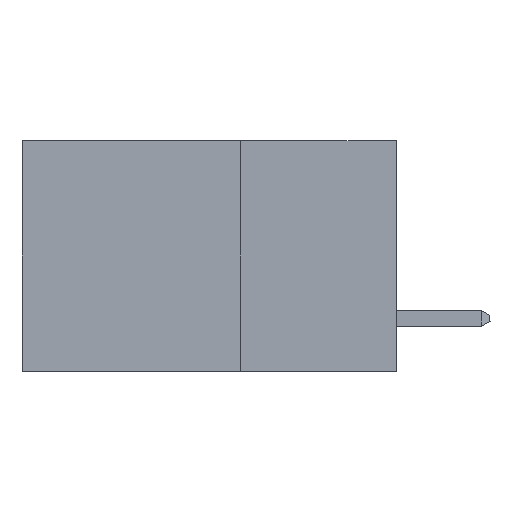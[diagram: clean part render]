
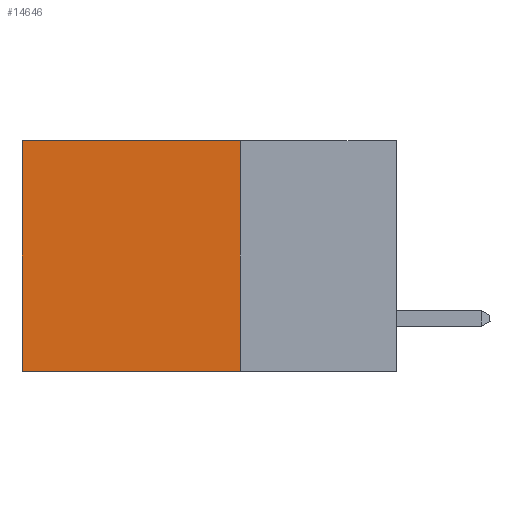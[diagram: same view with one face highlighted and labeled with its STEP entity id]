
A CAD part, left-side view. The second image highlights one B-rep face of the part: STEP entity #14646.
In plain terms, the highlighted planar face has unit normal (-1, 0, 0).
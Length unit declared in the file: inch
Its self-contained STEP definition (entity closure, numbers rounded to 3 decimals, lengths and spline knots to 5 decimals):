
#269 = LINE ( 'NONE', #2107, #10128 ) ;
#698 = CARTESIAN_POINT ( 'NONE',  ( 0.298, 0.6, 0. ) ) ;
#1136 = VECTOR ( 'NONE', #12388, 39.37008 ) ;
#1751 = VECTOR ( 'NONE', #14814, 39.37008 ) ;
#2107 = CARTESIAN_POINT ( 'NONE',  ( 0.298, 0.25, -0.37 ) ) ;
#2201 = ORIENTED_EDGE ( 'NONE', *, *, #11320, .T. ) ;
#3058 = CARTESIAN_POINT ( 'NONE',  ( 0.298, 0.25, 0. ) ) ;
#3590 = AXIS2_PLACEMENT_3D ( 'NONE', #3058, #5626, #14570 ) ;
#3721 = DIRECTION ( 'NONE',  ( 0., 0., -1. ) ) ;
#4056 = VERTEX_POINT ( 'NONE', #4396 ) ;
#4209 = EDGE_CURVE ( 'NONE', #4768, #14492, #8176, .T. ) ;
#4238 = EDGE_CURVE ( 'NONE', #4056, #7325, #4753, .T. ) ;
#4396 = CARTESIAN_POINT ( 'NONE',  ( 0.298, 0.25, 0. ) ) ;
#4753 = LINE ( 'NONE', #16504, #14184 ) ;
#4768 = VERTEX_POINT ( 'NONE', #11996 ) ;
#5626 = DIRECTION ( 'NONE',  ( 1., 0., 0. ) ) ;
#5871 = ORIENTED_EDGE ( 'NONE', *, *, #15448, .F. ) ;
#6697 = CARTESIAN_POINT ( 'NONE',  ( 0.298, 0.25, -0.37 ) ) ;
#7325 = VERTEX_POINT ( 'NONE', #6697 ) ;
#7377 = EDGE_LOOP ( 'NONE', ( #10195, #5871, #14433, #2201 ) ) ;
#7878 = CARTESIAN_POINT ( 'NONE',  ( 0.298, 0.6, -0.37 ) ) ;
#8176 = LINE ( 'NONE', #698, #1751 ) ;
#8550 = DIRECTION ( 'NONE',  ( 0., 1., 0. ) ) ;
#9761 = FACE_OUTER_BOUND ( 'NONE', #7377, .T. ) ;
#10128 = VECTOR ( 'NONE', #8550, 39.37008 ) ;
#10195 = ORIENTED_EDGE ( 'NONE', *, *, #4209, .T. ) ;
#11100 = CARTESIAN_POINT ( 'NONE',  ( 0.298, 0.25, 0. ) ) ;
#11320 = EDGE_CURVE ( 'NONE', #4056, #4768, #11381, .T. ) ;
#11381 = LINE ( 'NONE', #11100, #1136 ) ;
#11974 = PLANE ( 'NONE',  #3590 ) ;
#11996 = CARTESIAN_POINT ( 'NONE',  ( 0.298, 0.6, 0. ) ) ;
#12388 = DIRECTION ( 'NONE',  ( 0., 1., 0. ) ) ;
#14184 = VECTOR ( 'NONE', #3721, 39.37008 ) ;
#14433 = ORIENTED_EDGE ( 'NONE', *, *, #4238, .F. ) ;
#14492 = VERTEX_POINT ( 'NONE', #7878 ) ;
#14570 = DIRECTION ( 'NONE',  ( 0., 0., -1. ) ) ;
#14646 = ADVANCED_FACE ( 'NONE', ( #9761 ), #11974, .F. ) ;
#14814 = DIRECTION ( 'NONE',  ( 0., 0., -1. ) ) ;
#15448 = EDGE_CURVE ( 'NONE', #7325, #14492, #269, .T. ) ;
#16504 = CARTESIAN_POINT ( 'NONE',  ( 0.298, 0.25, 0. ) ) ;
